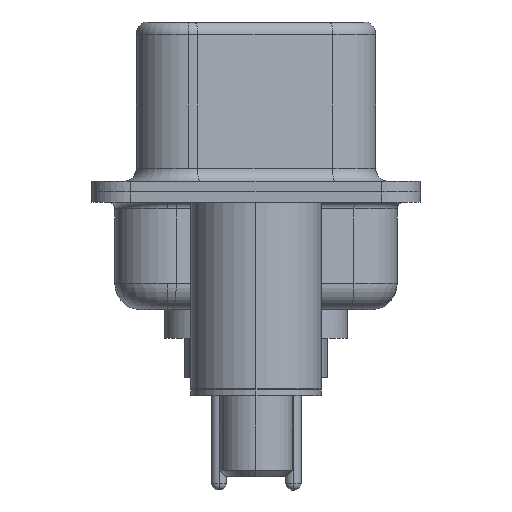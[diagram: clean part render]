
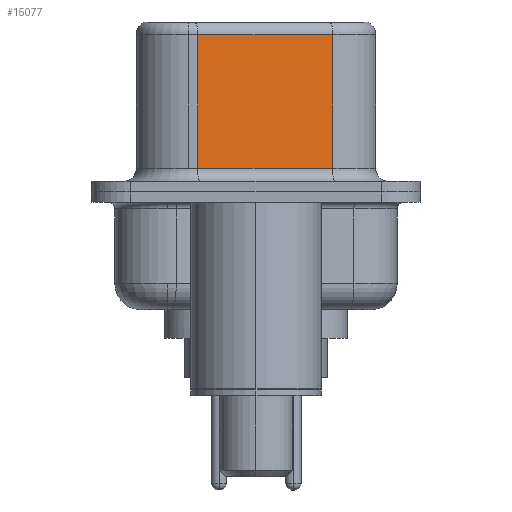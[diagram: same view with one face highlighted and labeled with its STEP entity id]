
A CAD part, left-side view. The second image highlights one B-rep face of the part: STEP entity #15077.
In plain terms, the highlighted planar face has unit normal (-0.985, -0.174, 0).
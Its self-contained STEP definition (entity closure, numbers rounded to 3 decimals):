
#462 = VERTEX_POINT ( 'NONE', #23397 ) ;
#886 = ORIENTED_EDGE ( 'NONE', *, *, #12940, .T. ) ;
#990 = CARTESIAN_POINT ( 'NONE',  ( 4.585, -2.927, 6.52 ) ) ;
#2795 = ORIENTED_EDGE ( 'NONE', *, *, #3326, .T. ) ;
#3326 = EDGE_CURVE ( 'NONE', #8353, #462, #4671, .T. ) ;
#4671 = LINE ( 'NONE', #19174, #13756 ) ;
#5855 = CARTESIAN_POINT ( 'NONE',  ( 4.585, -2.927, 6.52 ) ) ;
#5856 = VERTEX_POINT ( 'NONE', #23179 ) ;
#6197 = VERTEX_POINT ( 'NONE', #17831 ) ;
#6680 = EDGE_LOOP ( 'NONE', ( #14142, #18588, #886, #2795 ) ) ;
#8213 = LINE ( 'NONE', #5855, #22217 ) ;
#8285 = DIRECTION ( 'NONE',  ( 0.985, 0.174, 0. ) ) ;
#8353 = VERTEX_POINT ( 'NONE', #11549 ) ;
#9971 = FACE_OUTER_BOUND ( 'NONE', #6680, .T. ) ;
#10711 = EDGE_CURVE ( 'NONE', #6197, #5856, #18570, .T. ) ;
#11549 = CARTESIAN_POINT ( 'NONE',  ( 3.675, 2.233, 0.9 ) ) ;
#12940 = EDGE_CURVE ( 'NONE', #5856, #8353, #23551, .T. ) ;
#13706 = PLANE ( 'NONE',  #17961 ) ;
#13756 = VECTOR ( 'NONE', #18613, 1000. ) ;
#13791 = VECTOR ( 'NONE', #14478, 1000. ) ;
#14142 = ORIENTED_EDGE ( 'NONE', *, *, #17978, .F. ) ;
#14478 = DIRECTION ( 'NONE',  ( -0.174, 0.985, 0. ) ) ;
#15077 = ADVANCED_FACE ( 'NONE', ( #9971 ), #13706, .F. ) ;
#17242 = DIRECTION ( 'NONE',  ( 0., 0., -1. ) ) ;
#17831 = CARTESIAN_POINT ( 'NONE',  ( 4.585, -2.927, 6.02 ) ) ;
#17961 = AXIS2_PLACEMENT_3D ( 'NONE', #990, #8285, #21029 ) ;
#17978 = EDGE_CURVE ( 'NONE', #6197, #462, #8213, .T. ) ;
#18570 = LINE ( 'NONE', #19897, #13791 ) ;
#18588 = ORIENTED_EDGE ( 'NONE', *, *, #10711, .T. ) ;
#18613 = DIRECTION ( 'NONE',  ( 0.174, -0.985, 0. ) ) ;
#19039 = CARTESIAN_POINT ( 'NONE',  ( 3.675, 2.233, 6.52 ) ) ;
#19174 = CARTESIAN_POINT ( 'NONE',  ( 4.585, -2.927, 0.9 ) ) ;
#19897 = CARTESIAN_POINT ( 'NONE',  ( 4.585, -2.927, 6.02 ) ) ;
#21029 = DIRECTION ( 'NONE',  ( -0.174, 0.985, 0. ) ) ;
#21774 = VECTOR ( 'NONE', #17242, 1000. ) ;
#22217 = VECTOR ( 'NONE', #22314, 1000. ) ;
#22314 = DIRECTION ( 'NONE',  ( 0., 0., -1. ) ) ;
#23179 = CARTESIAN_POINT ( 'NONE',  ( 3.675, 2.233, 6.02 ) ) ;
#23397 = CARTESIAN_POINT ( 'NONE',  ( 4.585, -2.927, 0.9 ) ) ;
#23551 = LINE ( 'NONE', #19039, #21774 ) ;
